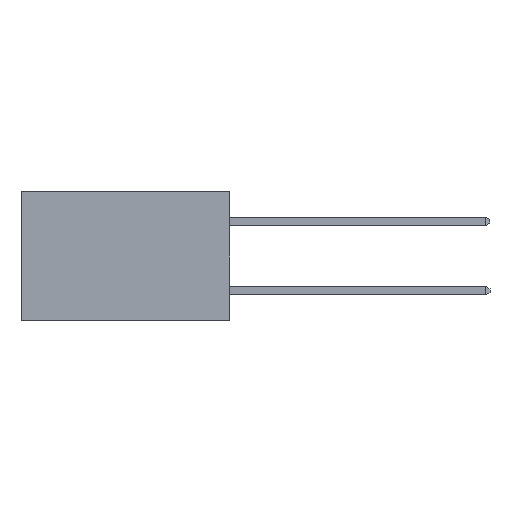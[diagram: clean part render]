
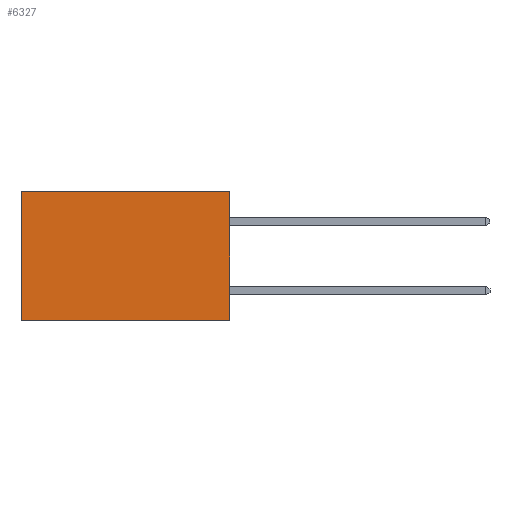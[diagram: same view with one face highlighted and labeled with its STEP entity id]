
A CAD part, left-side view. The second image highlights one B-rep face of the part: STEP entity #6327.
In plain terms, the highlighted planar face has unit normal (-1, 0, 0).
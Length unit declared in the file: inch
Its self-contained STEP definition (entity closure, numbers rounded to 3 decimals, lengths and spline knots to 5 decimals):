
#381 = EDGE_CURVE ( 'NONE', #8670, #768, #5134, .T. ) ;
#663 = FACE_OUTER_BOUND ( 'NONE', #1061, .T. ) ;
#768 = VERTEX_POINT ( 'NONE', #10193 ) ;
#894 = ORIENTED_EDGE ( 'NONE', *, *, #381, .F. ) ;
#1061 = EDGE_LOOP ( 'NONE', ( #2329, #2731, #894, #5236 ) ) ;
#2022 = CARTESIAN_POINT ( 'NONE',  ( 0.2615, 0., 0. ) ) ;
#2329 = ORIENTED_EDGE ( 'NONE', *, *, #6292, .T. ) ;
#2333 = AXIS2_PLACEMENT_3D ( 'NONE', #5147, #5086, #5052 ) ;
#2683 = CARTESIAN_POINT ( 'NONE',  ( 0.2615, 0., -0.37 ) ) ;
#2723 = DIRECTION ( 'NONE',  ( 0., 0., -1. ) ) ;
#2731 = ORIENTED_EDGE ( 'NONE', *, *, #6647, .F. ) ;
#3009 = VECTOR ( 'NONE', #2723, 39.37008 ) ;
#4422 = CARTESIAN_POINT ( 'NONE',  ( 0.2615, 0.6, -0.37 ) ) ;
#4791 = EDGE_CURVE ( 'NONE', #8670, #8870, #7415, .T. ) ;
#5052 = DIRECTION ( 'NONE',  ( 0., 0., -1. ) ) ;
#5086 = DIRECTION ( 'NONE',  ( 1., 0., 0. ) ) ;
#5134 = LINE ( 'NONE', #9942, #3009 ) ;
#5147 = CARTESIAN_POINT ( 'NONE',  ( 0.2615, 0., -0.37 ) ) ;
#5236 = ORIENTED_EDGE ( 'NONE', *, *, #4791, .T. ) ;
#5453 = PLANE ( 'NONE',  #2333 ) ;
#5534 = CARTESIAN_POINT ( 'NONE',  ( 0.2615, 0.6, -0.37 ) ) ;
#6060 = DIRECTION ( 'NONE',  ( 0., 0., -1. ) ) ;
#6292 = EDGE_CURVE ( 'NONE', #8870, #9568, #7982, .T. ) ;
#6327 = ADVANCED_FACE ( 'NONE', ( #663 ), #5453, .F. ) ;
#6360 = VECTOR ( 'NONE', #8342, 39.37008 ) ;
#6647 = EDGE_CURVE ( 'NONE', #768, #9568, #10156, .T. ) ;
#7058 = CARTESIAN_POINT ( 'NONE',  ( 0.2615, 0.6, 0. ) ) ;
#7127 = VECTOR ( 'NONE', #10308, 39.37008 ) ;
#7415 = LINE ( 'NONE', #10216, #7127 ) ;
#7982 = LINE ( 'NONE', #5534, #9258 ) ;
#8342 = DIRECTION ( 'NONE',  ( 0., 1., 0. ) ) ;
#8670 = VERTEX_POINT ( 'NONE', #2022 ) ;
#8870 = VERTEX_POINT ( 'NONE', #7058 ) ;
#9258 = VECTOR ( 'NONE', #6060, 39.37008 ) ;
#9568 = VERTEX_POINT ( 'NONE', #4422 ) ;
#9942 = CARTESIAN_POINT ( 'NONE',  ( 0.2615, 0., -0.37 ) ) ;
#10156 = LINE ( 'NONE', #2683, #6360 ) ;
#10193 = CARTESIAN_POINT ( 'NONE',  ( 0.2615, 0., -0.37 ) ) ;
#10216 = CARTESIAN_POINT ( 'NONE',  ( 0.2615, 0., 0. ) ) ;
#10308 = DIRECTION ( 'NONE',  ( 0., 1., 0. ) ) ;
